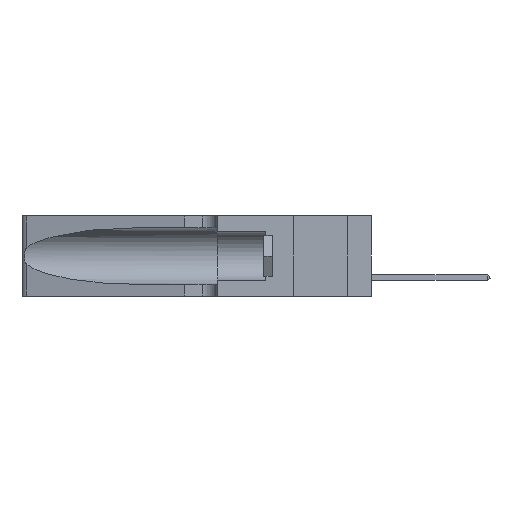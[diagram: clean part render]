
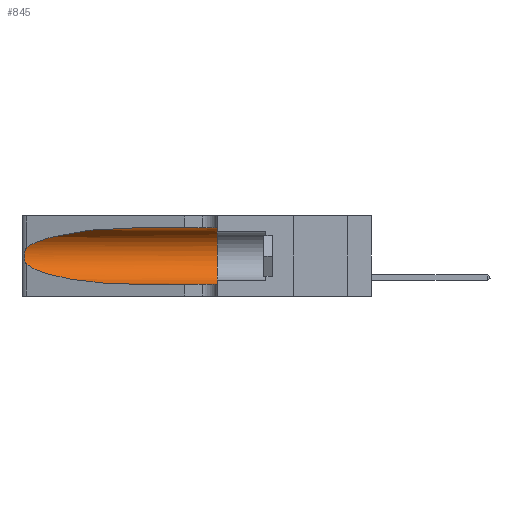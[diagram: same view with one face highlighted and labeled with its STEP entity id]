
A CAD part, left-side view. The second image highlights one B-rep face of the part: STEP entity #845.
In plain terms, the highlighted cylindrical face has radius 3.308 mm (diameter 6.617 mm), a partial arc.
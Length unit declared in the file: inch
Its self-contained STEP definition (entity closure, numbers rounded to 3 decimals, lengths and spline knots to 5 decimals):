
#69 = EDGE_CURVE ( 'NONE', #14071, #12508, #7555, .T. ) ;
#355 = AXIS2_PLACEMENT_3D ( 'NONE', #23505, #13428, #1481 ) ;
#646 = CARTESIAN_POINT ( 'NONE',  ( 0.1305, 0.72297, 0.05475 ) ) ;
#845 = ADVANCED_FACE ( 'NONE', ( #8205 ), #8510, .F. ) ;
#1322 = DIRECTION ( 'NONE',  ( 0., 0., 1. ) ) ;
#1481 = DIRECTION ( 'NONE',  ( 0., 0., -1. ) ) ;
#1693 = ORIENTED_EDGE ( 'NONE', *, *, #12938, .T. ) ;
#2654 = CARTESIAN_POINT ( 'NONE',  ( 0.25487, 1.22718, 0.14631 ) ) ;
#2714 = CARTESIAN_POINT ( 'NONE',  ( 0.26075, 1.23896, 0.178 ) ) ;
#2763 = B_SPLINE_CURVE_WITH_KNOTS ( 'NONE', 3,
 ( #25540, #13796, #15835, #3861, #11914, #5590, #12437, #2714, #6543, #10502, #24501, #8559, #15181, #7043 ),
 .UNSPECIFIED., .F., .F.,
 ( 4, 2, 2, 2, 2, 2, 4 ),
 ( 0., 0.00027, 0.00053, 0.00107, 0.0016, 0.00187, 0.00214 ),
 .UNSPECIFIED. ) ;
#3080 = DIRECTION ( 'NONE',  ( 0., 1., 0. ) ) ;
#3217 = CARTESIAN_POINT ( 'NONE',  ( 0.1305, 0.72297, 0.31525 ) ) ;
#3377 = CARTESIAN_POINT ( 'NONE',  ( 0.2373, 1.15595, 0.28018 ) ) ;
#3458 = CARTESIAN_POINT ( 'NONE',  ( 0.18966, 0.96281, 0.31525 ) ) ;
#3858 = CARTESIAN_POINT ( 'NONE',  ( 0.1305, 1.61858, 0.05475 ) ) ;
#3861 = CARTESIAN_POINT ( 'NONE',  ( 0.25787, 1.23484, 0.2124 ) ) ;
#4651 = CARTESIAN_POINT ( 'NONE',  ( 0.25487, 1.22718, 0.14631 ) ) ;
#5590 = CARTESIAN_POINT ( 'NONE',  ( 0.26018, 1.23835, 0.19895 ) ) ;
#5744 = EDGE_CURVE ( 'NONE', #17305, #12508, #23921, .T. ) ;
#5775 =( BOUNDED_CURVE ( )  B_SPLINE_CURVE ( 3, ( #2654, #22711, #16737, #6021 ),
 .UNSPECIFIED., .F., .F. ) 
 B_SPLINE_CURVE_WITH_KNOTS ( ( 4, 4 ),
 ( 3.44316, 4.71239 ),
 .UNSPECIFIED. ) 
 CURVE ( )  GEOMETRIC_REPRESENTATION_ITEM ( )  RATIONAL_B_SPLINE_CURVE ( ( 1., 0.87, 0.87, 1. ) ) 
 REPRESENTATION_ITEM ( '' )  );
#6021 = CARTESIAN_POINT ( 'NONE',  ( 0.1305, 0.72297, 0.05475 ) ) ;
#6271 =( BOUNDED_CURVE ( )  B_SPLINE_CURVE ( 3, ( #22898, #3458, #3377, #21608 ),
 .UNSPECIFIED., .F., .T. ) 
 B_SPLINE_CURVE_WITH_KNOTS ( ( 4, 4 ),
 ( 1.5708, 2.84003 ),
 .UNSPECIFIED. ) 
 CURVE ( )  GEOMETRIC_REPRESENTATION_ITEM ( )  RATIONAL_B_SPLINE_CURVE ( ( 1., 0.87, 0.87, 1. ) ) 
 REPRESENTATION_ITEM ( '' )  );
#6409 = EDGE_CURVE ( 'NONE', #16763, #17305, #5775, .T. ) ;
#6543 = CARTESIAN_POINT ( 'NONE',  ( 0.26017, 1.23833, 0.17102 ) ) ;
#7043 = CARTESIAN_POINT ( 'NONE',  ( 0.25487, 1.22718, 0.14631 ) ) ;
#7555 = CIRCLE ( 'NONE', #17795, 0.13025 ) ;
#7865 = ORIENTED_EDGE ( 'NONE', *, *, #6409, .T. ) ;
#8205 = FACE_OUTER_BOUND ( 'NONE', #17430, .T. ) ;
#8510 = CYLINDRICAL_SURFACE ( 'NONE', #355, 0.13025 ) ;
#8559 = CARTESIAN_POINT ( 'NONE',  ( 0.25639, 1.23186, 0.15144 ) ) ;
#9079 = LINE ( 'NONE', #17973, #24126 ) ;
#10477 = VECTOR ( 'NONE', #12350, 39.37008 ) ;
#10502 = CARTESIAN_POINT ( 'NONE',  ( 0.25856, 1.23593, 0.16098 ) ) ;
#11914 = CARTESIAN_POINT ( 'NONE',  ( 0.25854, 1.2359, 0.20912 ) ) ;
#12350 = DIRECTION ( 'NONE',  ( 0., -1., 0. ) ) ;
#12437 = CARTESIAN_POINT ( 'NONE',  ( 0.26075, 1.23896, 0.19203 ) ) ;
#12508 = VERTEX_POINT ( 'NONE', #18206 ) ;
#12938 = EDGE_CURVE ( 'NONE', #20236, #16763, #2763, .T. ) ;
#13428 = DIRECTION ( 'NONE',  ( 0., -1., 0. ) ) ;
#13796 = CARTESIAN_POINT ( 'NONE',  ( 0.25555, 1.22994, 0.2215 ) ) ;
#14071 = VERTEX_POINT ( 'NONE', #20841 ) ;
#15181 = CARTESIAN_POINT ( 'NONE',  ( 0.25555, 1.22993, 0.14849 ) ) ;
#15835 = CARTESIAN_POINT ( 'NONE',  ( 0.25639, 1.23184, 0.21858 ) ) ;
#16395 = ORIENTED_EDGE ( 'NONE', *, *, #24406, .F. ) ;
#16737 = CARTESIAN_POINT ( 'NONE',  ( 0.18966, 0.96281, 0.05475 ) ) ;
#16763 = VERTEX_POINT ( 'NONE', #4651 ) ;
#17305 = VERTEX_POINT ( 'NONE', #646 ) ;
#17430 = EDGE_LOOP ( 'NONE', ( #24591, #1693, #7865, #24303, #24565, #16395 ) ) ;
#17543 = EDGE_CURVE ( 'NONE', #19741, #20236, #6271, .T. ) ;
#17795 = AXIS2_PLACEMENT_3D ( 'NONE', #19290, #3080, #1322 ) ;
#17973 = CARTESIAN_POINT ( 'NONE',  ( 0.1305, 1.61858, 0.31525 ) ) ;
#18206 = CARTESIAN_POINT ( 'NONE',  ( 0.1305, 0.35, 0.05475 ) ) ;
#18911 = CARTESIAN_POINT ( 'NONE',  ( 0.25487, 1.22718, 0.22369 ) ) ;
#19290 = CARTESIAN_POINT ( 'NONE',  ( 0.1305, 0.35, 0.185 ) ) ;
#19741 = VERTEX_POINT ( 'NONE', #3217 ) ;
#20236 = VERTEX_POINT ( 'NONE', #18911 ) ;
#20841 = CARTESIAN_POINT ( 'NONE',  ( 0.1305, 0.35, 0.31525 ) ) ;
#21608 = CARTESIAN_POINT ( 'NONE',  ( 0.25487, 1.22718, 0.22369 ) ) ;
#22711 = CARTESIAN_POINT ( 'NONE',  ( 0.2373, 1.15595, 0.08982 ) ) ;
#22898 = CARTESIAN_POINT ( 'NONE',  ( 0.1305, 0.72297, 0.31525 ) ) ;
#23505 = CARTESIAN_POINT ( 'NONE',  ( 0.1305, 1.61858, 0.185 ) ) ;
#23921 = LINE ( 'NONE', #3858, #10477 ) ;
#24087 = DIRECTION ( 'NONE',  ( 0., -1., 0. ) ) ;
#24126 = VECTOR ( 'NONE', #24087, 39.37008 ) ;
#24303 = ORIENTED_EDGE ( 'NONE', *, *, #5744, .T. ) ;
#24406 = EDGE_CURVE ( 'NONE', #19741, #14071, #9079, .T. ) ;
#24501 = CARTESIAN_POINT ( 'NONE',  ( 0.25789, 1.23486, 0.15765 ) ) ;
#24565 = ORIENTED_EDGE ( 'NONE', *, *, #69, .F. ) ;
#24591 = ORIENTED_EDGE ( 'NONE', *, *, #17543, .T. ) ;
#25540 = CARTESIAN_POINT ( 'NONE',  ( 0.25487, 1.22718, 0.22369 ) ) ;
